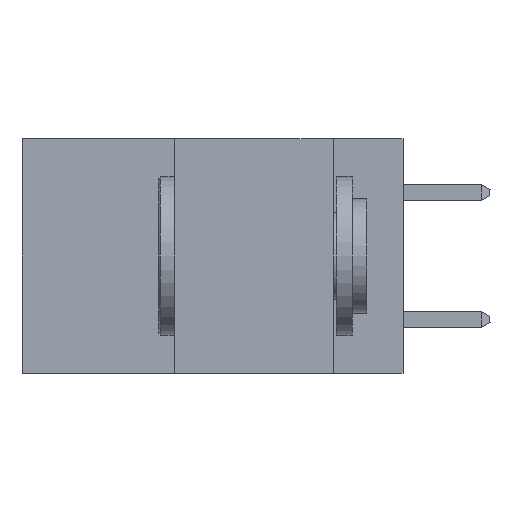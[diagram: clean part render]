
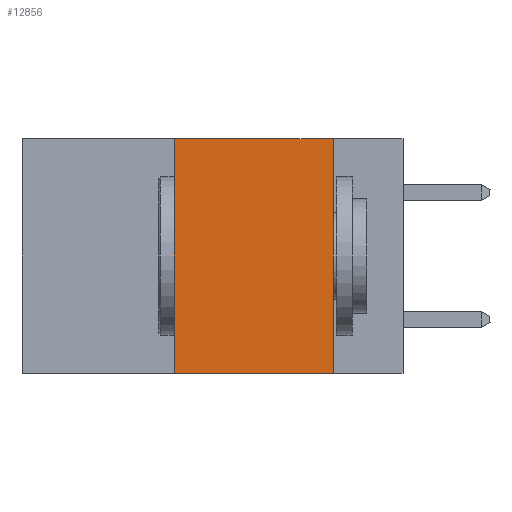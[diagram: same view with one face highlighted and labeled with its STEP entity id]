
A CAD part, left-side view. The second image highlights one B-rep face of the part: STEP entity #12856.
In plain terms, the highlighted planar face has unit normal (-1, 0, 0).
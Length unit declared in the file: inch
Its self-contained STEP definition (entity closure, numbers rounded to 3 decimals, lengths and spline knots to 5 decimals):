
#336 = AXIS2_PLACEMENT_3D ( 'NONE', #25759, #6749, #9149 ) ;
#382 = EDGE_CURVE ( 'NONE', #23277, #5870, #5907, .T. ) ;
#798 = FACE_OUTER_BOUND ( 'NONE', #11676, .T. ) ;
#3022 = DIRECTION ( 'NONE',  ( 0., -1., 0. ) ) ;
#4236 = ORIENTED_EDGE ( 'NONE', *, *, #23935, .F. ) ;
#4954 = ORIENTED_EDGE ( 'NONE', *, *, #382, .T. ) ;
#5013 = DIRECTION ( 'NONE',  ( 0., 0., -1. ) ) ;
#5187 = EDGE_CURVE ( 'NONE', #23457, #5870, #26706, .T. ) ;
#5322 = CARTESIAN_POINT ( 'NONE',  ( 0., 0.36, 0. ) ) ;
#5870 = VERTEX_POINT ( 'NONE', #17792 ) ;
#5886 = CARTESIAN_POINT ( 'NONE',  ( 0., 0.36, 0. ) ) ;
#5907 = LINE ( 'NONE', #8676, #16450 ) ;
#6749 = DIRECTION ( 'NONE',  ( 1., 0., 0. ) ) ;
#7954 = CARTESIAN_POINT ( 'NONE',  ( 0., 0.36, -0.37 ) ) ;
#8676 = CARTESIAN_POINT ( 'NONE',  ( 0., 0.6, -0.37 ) ) ;
#9149 = DIRECTION ( 'NONE',  ( 0., 0., -1. ) ) ;
#9601 = EDGE_CURVE ( 'NONE', #23277, #30832, #26923, .T. ) ;
#11676 = EDGE_LOOP ( 'NONE', ( #27342, #4236, #30375, #4954 ) ) ;
#12856 = ADVANCED_FACE ( 'NONE', ( #798 ), #21161, .F. ) ;
#14734 = CARTESIAN_POINT ( 'NONE',  ( 0., 0.6, 0. ) ) ;
#16450 = VECTOR ( 'NONE', #27884, 39.37008 ) ;
#16504 = CARTESIAN_POINT ( 'NONE',  ( 0., 0.11, 0. ) ) ;
#17792 = CARTESIAN_POINT ( 'NONE',  ( 0., 0.11, -0.37 ) ) ;
#20787 = VECTOR ( 'NONE', #5013, 39.37008 ) ;
#21161 = PLANE ( 'NONE',  #336 ) ;
#23277 = VERTEX_POINT ( 'NONE', #7954 ) ;
#23457 = VERTEX_POINT ( 'NONE', #30858 ) ;
#23935 = EDGE_CURVE ( 'NONE', #30832, #23457, #30652, .T. ) ;
#24370 = VECTOR ( 'NONE', #29727, 39.37008 ) ;
#25759 = CARTESIAN_POINT ( 'NONE',  ( 0., 0.6, 0. ) ) ;
#26706 = LINE ( 'NONE', #16504, #20787 ) ;
#26923 = LINE ( 'NONE', #5886, #24370 ) ;
#27342 = ORIENTED_EDGE ( 'NONE', *, *, #5187, .F. ) ;
#27884 = DIRECTION ( 'NONE',  ( 0., -1., 0. ) ) ;
#28008 = VECTOR ( 'NONE', #3022, 39.37008 ) ;
#29727 = DIRECTION ( 'NONE',  ( 0., 0., 1. ) ) ;
#30375 = ORIENTED_EDGE ( 'NONE', *, *, #9601, .F. ) ;
#30652 = LINE ( 'NONE', #14734, #28008 ) ;
#30832 = VERTEX_POINT ( 'NONE', #5322 ) ;
#30858 = CARTESIAN_POINT ( 'NONE',  ( 0., 0.11, 0. ) ) ;
